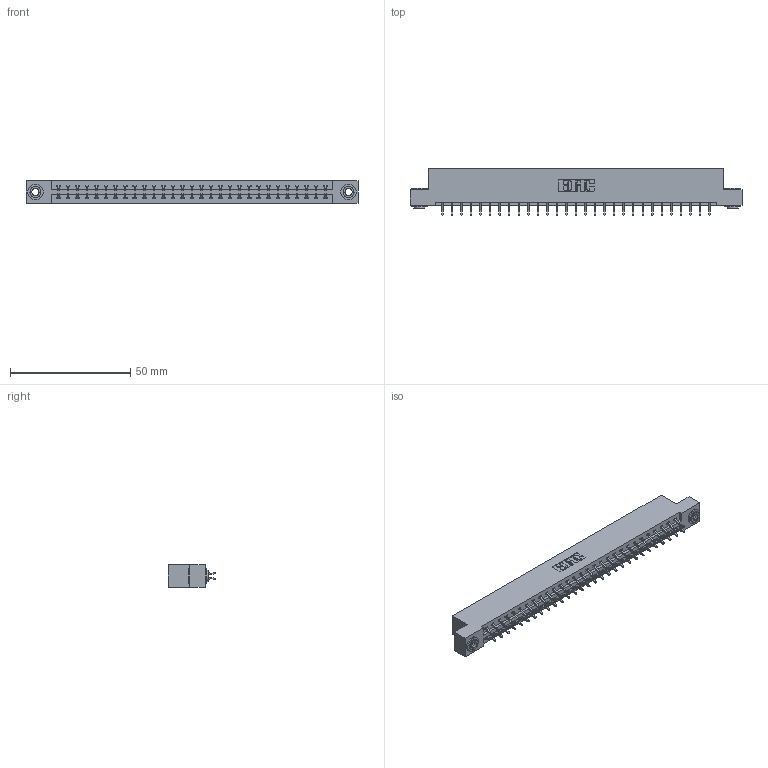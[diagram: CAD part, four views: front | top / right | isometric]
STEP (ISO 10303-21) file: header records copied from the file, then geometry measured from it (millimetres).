
FILE_DESCRIPTION (( 'STEP AP203' ), '1' );
FILE_NAME ('337-058-556-203.STEP', '2019-10-09T19:57:01', ( '' ), ( '' ), 'SwSTEP 2.0', 'SolidWorks 2016', '' );
FILE_SCHEMA (( 'CONFIG_CONTROL_DESIGN' ));
Length unit declared in the file: inch
Products named in the file (4): 337-058-556-203; 345-292-001_556 Tail; 337 Part_Flush Mounting Lugs - 0.156 Dia-TH; 345-250-002_345-250-002-102
Assembly tree (61 placements, depth 2):
  337-058-556-203
    337 Part_Flush Mounting Lugs - 0.156 Dia-TH
    345-292-001_556 Tail  x58
    345-250-002_345-250-002-102  x2
Bounding box: 137.92 x 19.57 x 9.4 mm (x, y, z)
Volume: 14379.4 mm3; surface area: 16292.8 mm2
Topology: 61 solids, 61 shells, 3632 faces, 10769 edges, 7098 vertices
Faces by surface type: plane 2516, cylinder 1108, cone 8
Entity records: 25036 total; most frequent: CARTESIAN_POINT 4217, ORIENTED_EDGE 4134, DIRECTION 3633, EDGE_CURVE 2067, LINE 1907, VECTOR 1907, VERTEX_POINT 1374, AXIS2_PLACEMENT_3D 863
